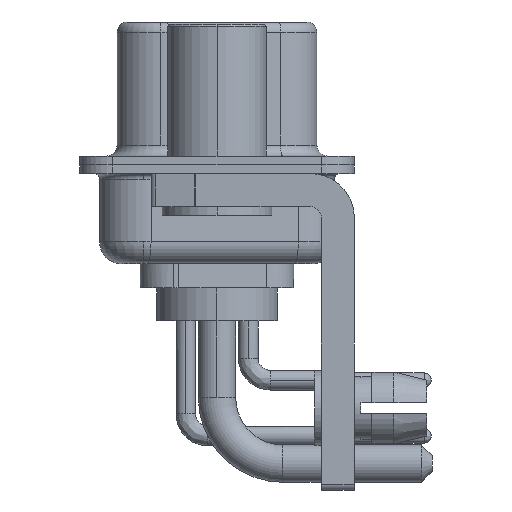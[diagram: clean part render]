
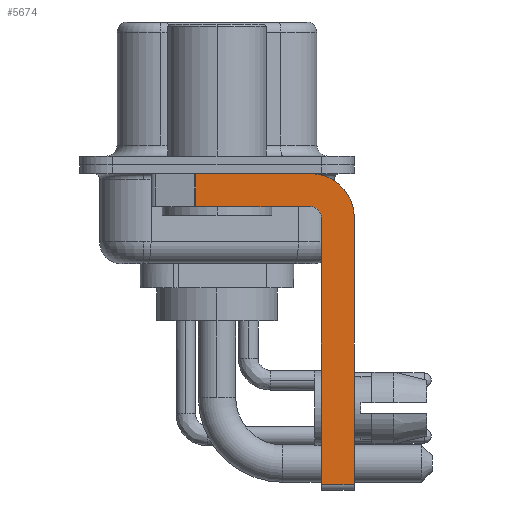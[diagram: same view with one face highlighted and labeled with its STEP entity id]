
A CAD part, left-side view. The second image highlights one B-rep face of the part: STEP entity #5674.
In plain terms, the highlighted planar face has unit normal (-1, 0, 0).
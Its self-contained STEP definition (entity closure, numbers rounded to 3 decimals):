
#118 = EDGE_CURVE ( 'NONE', #23139, #21921, #809, .T. ) ;
#161 = CARTESIAN_POINT ( 'NONE',  ( -2.9, -4.25, -1.9 ) ) ;
#222 = DIRECTION ( 'NONE',  ( 0., 0., -1. ) ) ;
#414 = AXIS2_PLACEMENT_3D ( 'NONE', #11109, #20272, #222 ) ;
#629 = EDGE_LOOP ( 'NONE', ( #24222, #13540, #17585, #16081, #13281, #16991, #5470, #27689 ) ) ;
#809 = LINE ( 'NONE', #13713, #10989 ) ;
#811 = VECTOR ( 'NONE', #1926, 1000. ) ;
#862 = VERTEX_POINT ( 'NONE', #15536 ) ;
#1161 = CARTESIAN_POINT ( 'NONE',  ( -2.9, -4.75, -2.4 ) ) ;
#1697 = DIRECTION ( 'NONE',  ( 0., 0., -1. ) ) ;
#1926 = DIRECTION ( 'NONE',  ( 0., 0., -1. ) ) ;
#3647 = LINE ( 'NONE', #21120, #811 ) ;
#4017 = VECTOR ( 'NONE', #25857, 1000. ) ;
#5470 = ORIENTED_EDGE ( 'NONE', *, *, #15657, .F. ) ;
#5625 = CARTESIAN_POINT ( 'NONE',  ( -2.9, -4.25, -2.4 ) ) ;
#5674 = ADVANCED_FACE ( 'NONE', ( #8822 ), #22409, .F. ) ;
#6607 = AXIS2_PLACEMENT_3D ( 'NONE', #16939, #27915, #14369 ) ;
#7052 = CIRCLE ( 'NONE', #6607, 0.5 ) ;
#7230 = VECTOR ( 'NONE', #23248, 1000. ) ;
#7799 = CARTESIAN_POINT ( 'NONE',  ( -2.9, 3., -0.4 ) ) ;
#8403 = CARTESIAN_POINT ( 'NONE',  ( -2.9, -4.25, -14.55 ) ) ;
#8822 = FACE_OUTER_BOUND ( 'NONE', #629, .T. ) ;
#8987 = VERTEX_POINT ( 'NONE', #16797 ) ;
#9840 = DIRECTION ( 'NONE',  ( 0., 0., 1. ) ) ;
#10874 = LINE ( 'NONE', #23886, #22273 ) ;
#10989 = VECTOR ( 'NONE', #9840, 1000. ) ;
#11109 = CARTESIAN_POINT ( 'NONE',  ( -2.9, -4.25, -2.4 ) ) ;
#11296 = VECTOR ( 'NONE', #1697, 1000. ) ;
#12158 = CARTESIAN_POINT ( 'NONE',  ( -2.9, -6.25, -14.55 ) ) ;
#12209 = DIRECTION ( 'NONE',  ( 0., 0., -1. ) ) ;
#12601 = EDGE_CURVE ( 'NONE', #21921, #17202, #7052, .T. ) ;
#13281 = ORIENTED_EDGE ( 'NONE', *, *, #118, .F. ) ;
#13540 = ORIENTED_EDGE ( 'NONE', *, *, #23446, .T. ) ;
#13713 = CARTESIAN_POINT ( 'NONE',  ( -2.9, -4.75, -14.8 ) ) ;
#13991 = CARTESIAN_POINT ( 'NONE',  ( -2.9, -4.25, -0.4 ) ) ;
#14137 = VERTEX_POINT ( 'NONE', #12158 ) ;
#14369 = DIRECTION ( 'NONE',  ( 0., 0., 1. ) ) ;
#14755 = LINE ( 'NONE', #23591, #11296 ) ;
#15536 = CARTESIAN_POINT ( 'NONE',  ( -2.9, -6.25, -2.4 ) ) ;
#15605 = DIRECTION ( 'NONE',  ( 0., 1., 0. ) ) ;
#15657 = EDGE_CURVE ( 'NONE', #862, #14137, #14755, .T. ) ;
#15806 = EDGE_CURVE ( 'NONE', #17202, #8987, #10874, .T. ) ;
#16038 = EDGE_CURVE ( 'NONE', #23139, #14137, #21586, .T. ) ;
#16081 = ORIENTED_EDGE ( 'NONE', *, *, #12601, .F. ) ;
#16516 = EDGE_CURVE ( 'NONE', #19448, #20704, #27385, .T. ) ;
#16797 = CARTESIAN_POINT ( 'NONE',  ( -2.9, 0.978, -1.9 ) ) ;
#16939 = CARTESIAN_POINT ( 'NONE',  ( -2.9, -4.25, -2.4 ) ) ;
#16991 = ORIENTED_EDGE ( 'NONE', *, *, #16038, .T. ) ;
#17202 = VERTEX_POINT ( 'NONE', #161 ) ;
#17585 = ORIENTED_EDGE ( 'NONE', *, *, #15806, .F. ) ;
#19448 = VERTEX_POINT ( 'NONE', #23102 ) ;
#20272 = DIRECTION ( 'NONE',  ( 1., 0., 0. ) ) ;
#20704 = VERTEX_POINT ( 'NONE', #13991 ) ;
#21120 = CARTESIAN_POINT ( 'NONE',  ( -2.9, 0.978, -1.9 ) ) ;
#21375 = DIRECTION ( 'NONE',  ( 1., 0., 0. ) ) ;
#21586 = LINE ( 'NONE', #8403, #4017 ) ;
#21921 = VERTEX_POINT ( 'NONE', #1161 ) ;
#22273 = VECTOR ( 'NONE', #15605, 1000. ) ;
#22409 = PLANE ( 'NONE',  #414 ) ;
#23102 = CARTESIAN_POINT ( 'NONE',  ( -2.9, 0.978, -0.4 ) ) ;
#23139 = VERTEX_POINT ( 'NONE', #26554 ) ;
#23248 = DIRECTION ( 'NONE',  ( 0., -1., 0. ) ) ;
#23446 = EDGE_CURVE ( 'NONE', #19448, #8987, #3647, .T. ) ;
#23591 = CARTESIAN_POINT ( 'NONE',  ( -2.9, -6.25, -2.4 ) ) ;
#23766 = CIRCLE ( 'NONE', #27859, 2. ) ;
#23886 = CARTESIAN_POINT ( 'NONE',  ( -2.9, -4.25, -1.9 ) ) ;
#24222 = ORIENTED_EDGE ( 'NONE', *, *, #16516, .F. ) ;
#25207 = EDGE_CURVE ( 'NONE', #20704, #862, #23766, .T. ) ;
#25857 = DIRECTION ( 'NONE',  ( 0., -1., 0. ) ) ;
#26554 = CARTESIAN_POINT ( 'NONE',  ( -2.9, -4.75, -14.55 ) ) ;
#27385 = LINE ( 'NONE', #7799, #7230 ) ;
#27689 = ORIENTED_EDGE ( 'NONE', *, *, #25207, .F. ) ;
#27859 = AXIS2_PLACEMENT_3D ( 'NONE', #5625, #21375, #12209 ) ;
#27915 = DIRECTION ( 'NONE',  ( -1., 0., 0. ) ) ;
